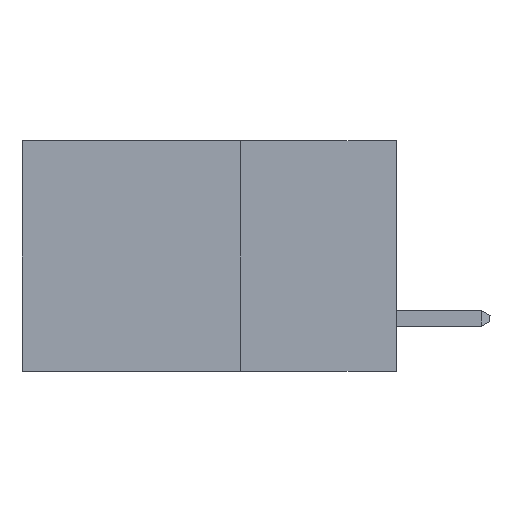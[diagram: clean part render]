
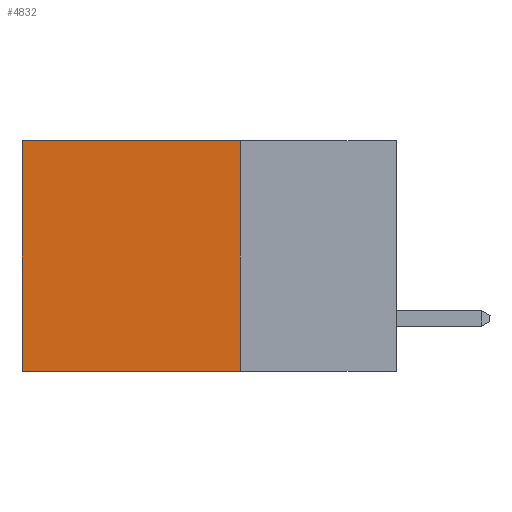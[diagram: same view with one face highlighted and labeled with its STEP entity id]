
A CAD part, left-side view. The second image highlights one B-rep face of the part: STEP entity #4832.
In plain terms, the highlighted planar face has unit normal (-1, 0, 0).
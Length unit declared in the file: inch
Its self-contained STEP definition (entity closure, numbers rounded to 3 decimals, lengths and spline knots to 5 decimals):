
#376 = CARTESIAN_POINT ( 'NONE',  ( 0.2615, 0.25, 0. ) ) ;
#622 = CARTESIAN_POINT ( 'NONE',  ( 0.2615, 0.25, -0.37 ) ) ;
#672 = AXIS2_PLACEMENT_3D ( 'NONE', #1361, #6588, #7863 ) ;
#945 = VERTEX_POINT ( 'NONE', #376 ) ;
#1230 = EDGE_LOOP ( 'NONE', ( #6464, #4626, #3649, #3166 ) ) ;
#1361 = CARTESIAN_POINT ( 'NONE',  ( 0.2615, 0.25, -0.37 ) ) ;
#1579 = CARTESIAN_POINT ( 'NONE',  ( 0.2615, 0.25, -0.37 ) ) ;
#2845 = LINE ( 'NONE', #5041, #6421 ) ;
#3077 = CARTESIAN_POINT ( 'NONE',  ( 0.2615, 0.6, -0.37 ) ) ;
#3166 = ORIENTED_EDGE ( 'NONE', *, *, #10839, .T. ) ;
#3256 = VECTOR ( 'NONE', #4272, 39.37008 ) ;
#3649 = ORIENTED_EDGE ( 'NONE', *, *, #11223, .F. ) ;
#3656 = DIRECTION ( 'NONE',  ( 0., 1., 0. ) ) ;
#3862 = LINE ( 'NONE', #622, #13661 ) ;
#3980 = DIRECTION ( 'NONE',  ( 0., 0., -1. ) ) ;
#4272 = DIRECTION ( 'NONE',  ( 0., 1., 0. ) ) ;
#4626 = ORIENTED_EDGE ( 'NONE', *, *, #9326, .F. ) ;
#4709 = VECTOR ( 'NONE', #8982, 39.37008 ) ;
#4750 = LINE ( 'NONE', #9046, #4709 ) ;
#4832 = ADVANCED_FACE ( 'NONE', ( #9810 ), #12119, .F. ) ;
#5041 = CARTESIAN_POINT ( 'NONE',  ( 0.2615, 0.25, -0.37 ) ) ;
#5336 = LINE ( 'NONE', #11763, #3256 ) ;
#6421 = VECTOR ( 'NONE', #3980, 39.37008 ) ;
#6464 = ORIENTED_EDGE ( 'NONE', *, *, #9562, .T. ) ;
#6588 = DIRECTION ( 'NONE',  ( 1., 0., 0. ) ) ;
#7863 = DIRECTION ( 'NONE',  ( 0., 0., -1. ) ) ;
#8982 = DIRECTION ( 'NONE',  ( 0., 0., -1. ) ) ;
#9046 = CARTESIAN_POINT ( 'NONE',  ( 0.2615, 0.6, -0.37 ) ) ;
#9326 = EDGE_CURVE ( 'NONE', #11034, #13241, #3862, .T. ) ;
#9562 = EDGE_CURVE ( 'NONE', #13096, #13241, #4750, .T. ) ;
#9810 = FACE_OUTER_BOUND ( 'NONE', #1230, .T. ) ;
#10839 = EDGE_CURVE ( 'NONE', #945, #13096, #5336, .T. ) ;
#11034 = VERTEX_POINT ( 'NONE', #1579 ) ;
#11223 = EDGE_CURVE ( 'NONE', #945, #11034, #2845, .T. ) ;
#11763 = CARTESIAN_POINT ( 'NONE',  ( 0.2615, 0.25, 0. ) ) ;
#12119 = PLANE ( 'NONE',  #672 ) ;
#13077 = CARTESIAN_POINT ( 'NONE',  ( 0.2615, 0.6, 0. ) ) ;
#13096 = VERTEX_POINT ( 'NONE', #13077 ) ;
#13241 = VERTEX_POINT ( 'NONE', #3077 ) ;
#13661 = VECTOR ( 'NONE', #3656, 39.37008 ) ;
